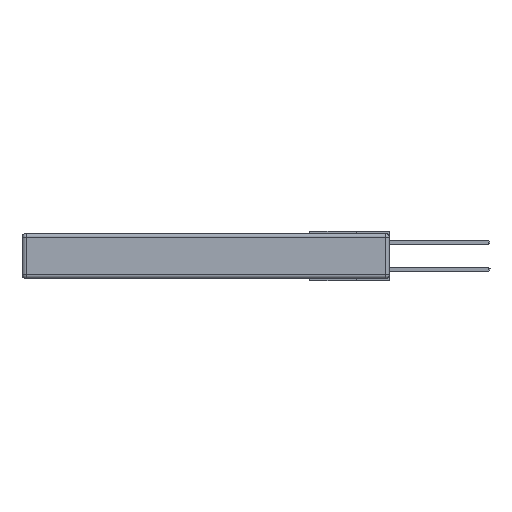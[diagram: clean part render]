
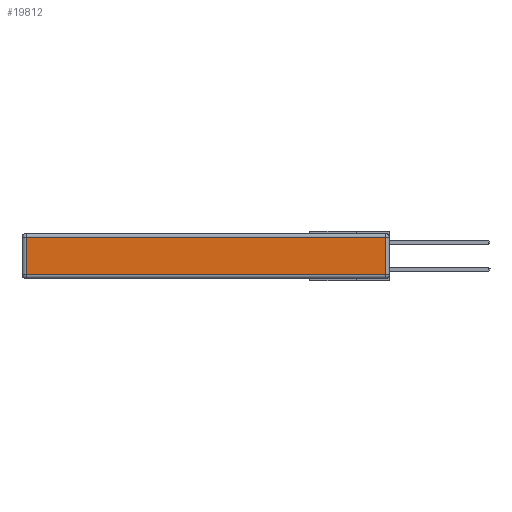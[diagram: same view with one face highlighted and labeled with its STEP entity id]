
A CAD part, left-side view. The second image highlights one B-rep face of the part: STEP entity #19812.
In plain terms, the highlighted planar face has unit normal (-1, 0, 0).
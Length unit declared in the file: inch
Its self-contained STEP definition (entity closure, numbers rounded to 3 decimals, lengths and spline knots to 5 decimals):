
#342 = CARTESIAN_POINT ( 'NONE',  ( 0., 2.72, -0.343 ) ) ;
#595 = EDGE_CURVE ( 'NONE', #13635, #4661, #15365, .T. ) ;
#649 = DIRECTION ( 'NONE',  ( 0., 0., 1. ) ) ;
#1557 = AXIS2_PLACEMENT_3D ( 'NONE', #22228, #26190, #3248 ) ;
#3248 = DIRECTION ( 'NONE',  ( 0., 0., 1. ) ) ;
#3752 = CARTESIAN_POINT ( 'NONE',  ( 0., 0.03, -0.03 ) ) ;
#4466 = CARTESIAN_POINT ( 'NONE',  ( 0., 2.72, -0.03 ) ) ;
#4622 = CARTESIAN_POINT ( 'NONE',  ( 0., 0.03, -0.343 ) ) ;
#4661 = VERTEX_POINT ( 'NONE', #3752 ) ;
#5439 = LINE ( 'NONE', #22415, #14075 ) ;
#8137 = FACE_OUTER_BOUND ( 'NONE', #24161, .T. ) ;
#11513 = PLANE ( 'NONE',  #1557 ) ;
#12002 = EDGE_CURVE ( 'NONE', #4661, #25621, #5439, .T. ) ;
#12461 = DIRECTION ( 'NONE',  ( 0., -1., 0. ) ) ;
#12573 = VECTOR ( 'NONE', #16916, 39.37008 ) ;
#13200 = LINE ( 'NONE', #342, #12573 ) ;
#13502 = ORIENTED_EDGE ( 'NONE', *, *, #15139, .T. ) ;
#13586 = ORIENTED_EDGE ( 'NONE', *, *, #12002, .T. ) ;
#13635 = VERTEX_POINT ( 'NONE', #15558 ) ;
#14026 = ORIENTED_EDGE ( 'NONE', *, *, #21397, .T. ) ;
#14075 = VECTOR ( 'NONE', #24293, 39.37008 ) ;
#15139 = EDGE_CURVE ( 'NONE', #23230, #13635, #21735, .T. ) ;
#15365 = LINE ( 'NONE', #4622, #18602 ) ;
#15558 = CARTESIAN_POINT ( 'NONE',  ( 0., 0.03, -0.313 ) ) ;
#16916 = DIRECTION ( 'NONE',  ( 0., 0., -1. ) ) ;
#18491 = VECTOR ( 'NONE', #12461, 39.37008 ) ;
#18602 = VECTOR ( 'NONE', #649, 39.37008 ) ;
#19708 = ORIENTED_EDGE ( 'NONE', *, *, #595, .T. ) ;
#19812 = ADVANCED_FACE ( 'NONE', ( #8137 ), #11513, .T. ) ;
#21397 = EDGE_CURVE ( 'NONE', #25621, #23230, #13200, .T. ) ;
#21735 = LINE ( 'NONE', #24465, #18491 ) ;
#22022 = CARTESIAN_POINT ( 'NONE',  ( 0., 2.72, -0.313 ) ) ;
#22228 = CARTESIAN_POINT ( 'NONE',  ( 0., 0., -0.343 ) ) ;
#22415 = CARTESIAN_POINT ( 'NONE',  ( 0., 2.75, -0.03 ) ) ;
#23230 = VERTEX_POINT ( 'NONE', #22022 ) ;
#24161 = EDGE_LOOP ( 'NONE', ( #13502, #19708, #13586, #14026 ) ) ;
#24293 = DIRECTION ( 'NONE',  ( 0., 1., 0. ) ) ;
#24465 = CARTESIAN_POINT ( 'NONE',  ( 0., 0., -0.313 ) ) ;
#25621 = VERTEX_POINT ( 'NONE', #4466 ) ;
#26190 = DIRECTION ( 'NONE',  ( -1., 0., 0. ) ) ;
